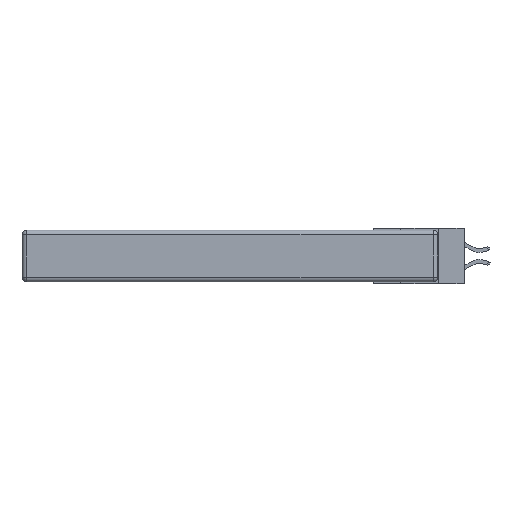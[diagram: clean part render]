
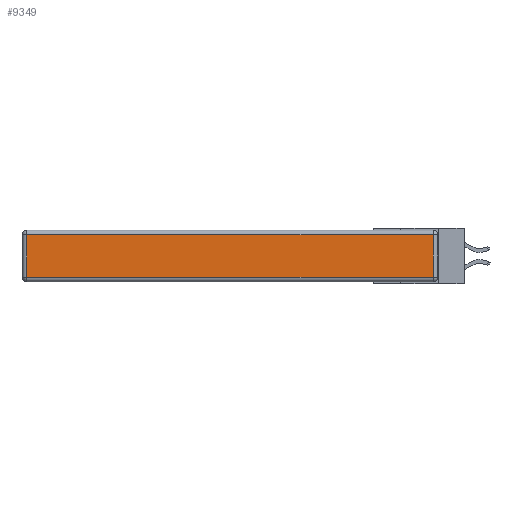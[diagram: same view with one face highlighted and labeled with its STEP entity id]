
A CAD part, left-side view. The second image highlights one B-rep face of the part: STEP entity #9349.
In plain terms, the highlighted planar face has unit normal (-1, 0, 0).
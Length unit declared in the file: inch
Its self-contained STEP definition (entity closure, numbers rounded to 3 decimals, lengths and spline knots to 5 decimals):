
#1 = CARTESIAN_POINT ( 'NONE',  ( 0., 0.03, -0.343 ) ) ;
#76 = ORIENTED_EDGE ( 'NONE', *, *, #2503, .T. ) ;
#678 = DIRECTION ( 'NONE',  ( 0., -1., 0. ) ) ;
#984 = VECTOR ( 'NONE', #678, 39.37008 ) ;
#1267 = DIRECTION ( 'NONE',  ( -1., 0., 0. ) ) ;
#1585 = ORIENTED_EDGE ( 'NONE', *, *, #5485, .T. ) ;
#1933 = CARTESIAN_POINT ( 'NONE',  ( 0., 0., -0.313 ) ) ;
#1952 = VERTEX_POINT ( 'NONE', #2924 ) ;
#2503 = EDGE_CURVE ( 'NONE', #9823, #4100, #10206, .T. ) ;
#2924 = CARTESIAN_POINT ( 'NONE',  ( 0., 2.72, -0.313 ) ) ;
#3779 = DIRECTION ( 'NONE',  ( 0., 0., 1. ) ) ;
#4100 = VERTEX_POINT ( 'NONE', #8778 ) ;
#4127 = CARTESIAN_POINT ( 'NONE',  ( 0., 0.03, -0.313 ) ) ;
#4840 = ORIENTED_EDGE ( 'NONE', *, *, #6619, .T. ) ;
#5123 = PLANE ( 'NONE',  #6204 ) ;
#5485 = EDGE_CURVE ( 'NONE', #4100, #1952, #12475, .T. ) ;
#5990 = CARTESIAN_POINT ( 'NONE',  ( 0., 0.03, -0.03 ) ) ;
#6204 = AXIS2_PLACEMENT_3D ( 'NONE', #13957, #1267, #3779 ) ;
#6619 = EDGE_CURVE ( 'NONE', #7256, #9823, #12638, .T. ) ;
#6799 = CARTESIAN_POINT ( 'NONE',  ( 0., 2.72, -0.343 ) ) ;
#6899 = DIRECTION ( 'NONE',  ( 0., 0., -1. ) ) ;
#7256 = VERTEX_POINT ( 'NONE', #4127 ) ;
#7313 = EDGE_CURVE ( 'NONE', #1952, #7256, #12824, .T. ) ;
#7452 = EDGE_LOOP ( 'NONE', ( #10997, #4840, #76, #1585 ) ) ;
#8778 = CARTESIAN_POINT ( 'NONE',  ( 0., 2.72, -0.03 ) ) ;
#9265 = VECTOR ( 'NONE', #12549, 39.37008 ) ;
#9349 = ADVANCED_FACE ( 'NONE', ( #14941 ), #5123, .T. ) ;
#9823 = VERTEX_POINT ( 'NONE', #5990 ) ;
#10206 = LINE ( 'NONE', #16225, #16122 ) ;
#10997 = ORIENTED_EDGE ( 'NONE', *, *, #7313, .T. ) ;
#12468 = DIRECTION ( 'NONE',  ( 0., 1., 0. ) ) ;
#12475 = LINE ( 'NONE', #6799, #16234 ) ;
#12549 = DIRECTION ( 'NONE',  ( 0., 0., 1. ) ) ;
#12638 = LINE ( 'NONE', #1, #9265 ) ;
#12824 = LINE ( 'NONE', #1933, #984 ) ;
#13957 = CARTESIAN_POINT ( 'NONE',  ( 0., 0., -0.343 ) ) ;
#14941 = FACE_OUTER_BOUND ( 'NONE', #7452, .T. ) ;
#16122 = VECTOR ( 'NONE', #12468, 39.37008 ) ;
#16225 = CARTESIAN_POINT ( 'NONE',  ( 0., 2.75, -0.03 ) ) ;
#16234 = VECTOR ( 'NONE', #6899, 39.37008 ) ;
